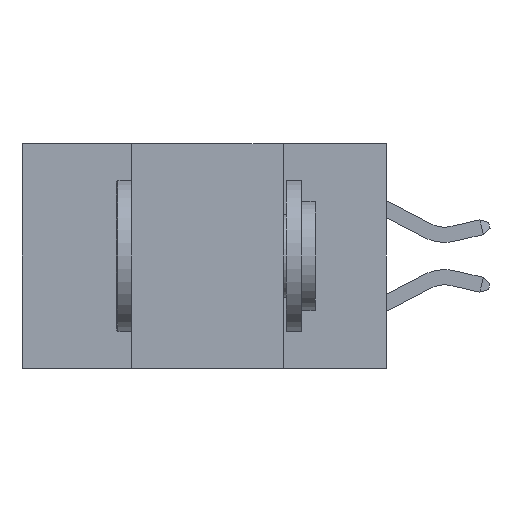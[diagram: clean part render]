
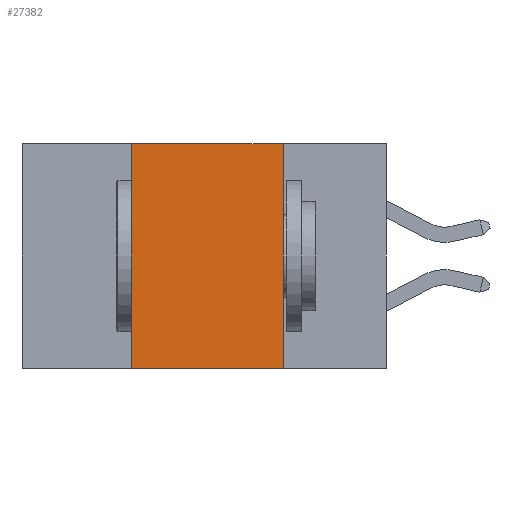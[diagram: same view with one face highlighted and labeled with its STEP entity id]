
A CAD part, left-side view. The second image highlights one B-rep face of the part: STEP entity #27382.
In plain terms, the highlighted planar face has unit normal (-1, 0, 0).
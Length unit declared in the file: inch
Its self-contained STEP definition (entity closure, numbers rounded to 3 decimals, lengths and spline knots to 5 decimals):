
#409 = VERTEX_POINT ( 'NONE', #959 ) ;
#896 = VECTOR ( 'NONE', #12842, 39.37008 ) ;
#959 = CARTESIAN_POINT ( 'NONE',  ( 0., 0.17, -0.37 ) ) ;
#2847 = CARTESIAN_POINT ( 'NONE',  ( 0., 0.6, -0.37 ) ) ;
#2950 = LINE ( 'NONE', #15396, #19187 ) ;
#3085 = VERTEX_POINT ( 'NONE', #10369 ) ;
#4839 = ORIENTED_EDGE ( 'NONE', *, *, #18876, .F. ) ;
#4923 = DIRECTION ( 'NONE',  ( 0., -1., 0. ) ) ;
#6504 = PLANE ( 'NONE',  #22366 ) ;
#8018 = EDGE_CURVE ( 'NONE', #24128, #409, #18567, .T. ) ;
#9073 = LINE ( 'NONE', #2847, #25852 ) ;
#10369 = CARTESIAN_POINT ( 'NONE',  ( 0., 0.42, 0. ) ) ;
#10647 = EDGE_LOOP ( 'NONE', ( #13239, #26137, #4839, #15664 ) ) ;
#11112 = DIRECTION ( 'NONE',  ( 0., 0., -1. ) ) ;
#12126 = LINE ( 'NONE', #24732, #23054 ) ;
#12842 = DIRECTION ( 'NONE',  ( 0., 0., -1. ) ) ;
#12974 = CARTESIAN_POINT ( 'NONE',  ( 0., 0.17, 0. ) ) ;
#13239 = ORIENTED_EDGE ( 'NONE', *, *, #8018, .F. ) ;
#13725 = CARTESIAN_POINT ( 'NONE',  ( 0., 0.17, 0. ) ) ;
#15396 = CARTESIAN_POINT ( 'NONE',  ( 0., 0.42, 0. ) ) ;
#15664 = ORIENTED_EDGE ( 'NONE', *, *, #26056, .T. ) ;
#17621 = DIRECTION ( 'NONE',  ( 0., 0., 1. ) ) ;
#18567 = LINE ( 'NONE', #12974, #896 ) ;
#18876 = EDGE_CURVE ( 'NONE', #25934, #3085, #2950, .T. ) ;
#19187 = VECTOR ( 'NONE', #17621, 39.37008 ) ;
#19746 = FACE_OUTER_BOUND ( 'NONE', #10647, .T. ) ;
#19849 = CARTESIAN_POINT ( 'NONE',  ( 0., 0.6, 0. ) ) ;
#20013 = CARTESIAN_POINT ( 'NONE',  ( 0., 0.42, -0.37 ) ) ;
#22366 = AXIS2_PLACEMENT_3D ( 'NONE', #19849, #24199, #11112 ) ;
#22537 = EDGE_CURVE ( 'NONE', #3085, #24128, #12126, .T. ) ;
#23054 = VECTOR ( 'NONE', #26814, 39.37008 ) ;
#24128 = VERTEX_POINT ( 'NONE', #13725 ) ;
#24199 = DIRECTION ( 'NONE',  ( 1., 0., 0. ) ) ;
#24732 = CARTESIAN_POINT ( 'NONE',  ( 0., 0.6, 0. ) ) ;
#25852 = VECTOR ( 'NONE', #4923, 39.37008 ) ;
#25934 = VERTEX_POINT ( 'NONE', #20013 ) ;
#26056 = EDGE_CURVE ( 'NONE', #25934, #409, #9073, .T. ) ;
#26137 = ORIENTED_EDGE ( 'NONE', *, *, #22537, .F. ) ;
#26814 = DIRECTION ( 'NONE',  ( 0., -1., 0. ) ) ;
#27382 = ADVANCED_FACE ( 'NONE', ( #19746 ), #6504, .F. ) ;
